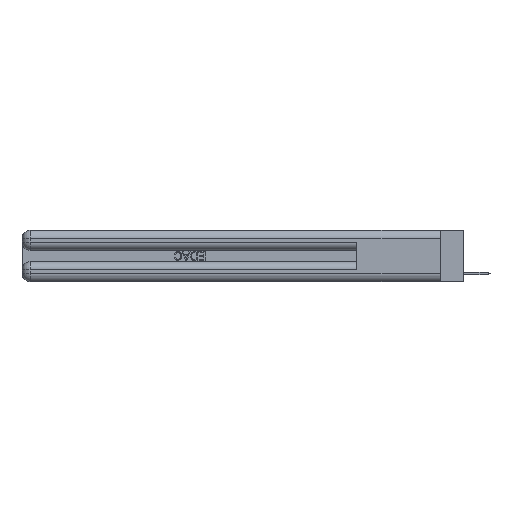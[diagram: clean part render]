
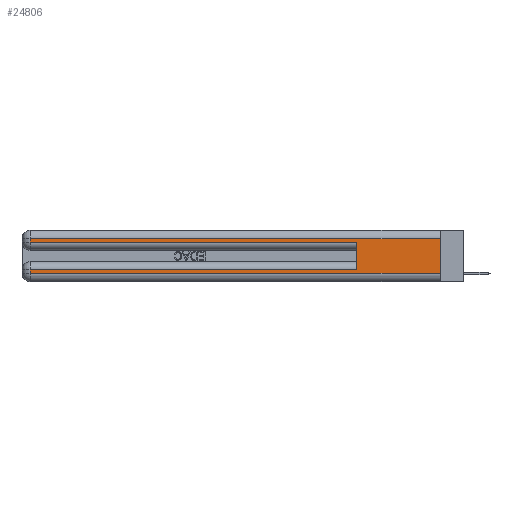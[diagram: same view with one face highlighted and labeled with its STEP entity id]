
A CAD part, left-side view. The second image highlights one B-rep face of the part: STEP entity #24806.
In plain terms, the highlighted planar face has unit normal (-1, 0, 0).
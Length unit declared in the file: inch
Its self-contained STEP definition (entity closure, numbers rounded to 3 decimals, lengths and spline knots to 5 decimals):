
#79 = VECTOR ( 'NONE', #12327, 39.37008 ) ;
#228 = DIRECTION ( 'NONE',  ( 0., 0., -1. ) ) ;
#763 = LINE ( 'NONE', #18012, #22861 ) ;
#814 = CARTESIAN_POINT ( 'NONE',  ( 0., 0.6, 0.285 ) ) ;
#931 = CARTESIAN_POINT ( 'NONE',  ( 0., 2.94, 0.31 ) ) ;
#2115 = ORIENTED_EDGE ( 'NONE', *, *, #25641, .T. ) ;
#2352 = LINE ( 'NONE', #28300, #20091 ) ;
#2500 = CARTESIAN_POINT ( 'NONE',  ( 0., 0., 0.085 ) ) ;
#2709 = ORIENTED_EDGE ( 'NONE', *, *, #18675, .T. ) ;
#3189 = DIRECTION ( 'NONE',  ( 0., 0., -1. ) ) ;
#3771 = DIRECTION ( 'NONE',  ( 0., -1., 0. ) ) ;
#4194 = LINE ( 'NONE', #7821, #12872 ) ;
#5015 = DIRECTION ( 'NONE',  ( 0., 0., -1. ) ) ;
#5407 = PLANE ( 'NONE',  #27420 ) ;
#5705 = CARTESIAN_POINT ( 'NONE',  ( 0., 0., 0.37 ) ) ;
#5815 = VERTEX_POINT ( 'NONE', #12371 ) ;
#6449 = VERTEX_POINT ( 'NONE', #814 ) ;
#6516 = EDGE_CURVE ( 'NONE', #10701, #6449, #26906, .T. ) ;
#7080 = VECTOR ( 'NONE', #3771, 39.37008 ) ;
#7821 = CARTESIAN_POINT ( 'NONE',  ( 0., 0., 0.31 ) ) ;
#8085 = EDGE_CURVE ( 'NONE', #5815, #6449, #763, .T. ) ;
#8103 = VERTEX_POINT ( 'NONE', #27344 ) ;
#8982 = CARTESIAN_POINT ( 'NONE',  ( 0., 2.94, 0.06 ) ) ;
#9684 = ORIENTED_EDGE ( 'NONE', *, *, #15189, .F. ) ;
#10701 = VERTEX_POINT ( 'NONE', #14989 ) ;
#12074 = CARTESIAN_POINT ( 'NONE',  ( 0., 0., 0.31 ) ) ;
#12327 = DIRECTION ( 'NONE',  ( 0., 0., 1. ) ) ;
#12371 = CARTESIAN_POINT ( 'NONE',  ( 0., 2.94, 0.285 ) ) ;
#12578 = DIRECTION ( 'NONE',  ( 1., 0., 0. ) ) ;
#12631 = CARTESIAN_POINT ( 'NONE',  ( 0., 0.6, 0.145 ) ) ;
#12872 = VECTOR ( 'NONE', #23879, 39.37008 ) ;
#13074 = CARTESIAN_POINT ( 'NONE',  ( 0., 0., 0.37 ) ) ;
#13651 = EDGE_CURVE ( 'NONE', #27425, #5815, #22936, .T. ) ;
#14601 = VECTOR ( 'NONE', #228, 39.37008 ) ;
#14660 = ORIENTED_EDGE ( 'NONE', *, *, #19302, .T. ) ;
#14989 = CARTESIAN_POINT ( 'NONE',  ( 0., 0.6, 0.085 ) ) ;
#15189 = EDGE_CURVE ( 'NONE', #16778, #8103, #27572, .T. ) ;
#15810 = FACE_OUTER_BOUND ( 'NONE', #24978, .T. ) ;
#16471 = LINE ( 'NONE', #17611, #7080 ) ;
#16706 = VECTOR ( 'NONE', #29312, 39.37008 ) ;
#16778 = VERTEX_POINT ( 'NONE', #12074 ) ;
#17611 = CARTESIAN_POINT ( 'NONE',  ( 0., 0., 0.06 ) ) ;
#17873 = VERTEX_POINT ( 'NONE', #18712 ) ;
#18012 = CARTESIAN_POINT ( 'NONE',  ( 0., 0., 0.285 ) ) ;
#18585 = VECTOR ( 'NONE', #25759, 39.37008 ) ;
#18675 = EDGE_CURVE ( 'NONE', #16778, #27425, #4194, .T. ) ;
#18712 = CARTESIAN_POINT ( 'NONE',  ( 0., 2.94, 0.085 ) ) ;
#19184 = ORIENTED_EDGE ( 'NONE', *, *, #8085, .T. ) ;
#19302 = EDGE_CURVE ( 'NONE', #17873, #21687, #2352, .T. ) ;
#20091 = VECTOR ( 'NONE', #5015, 39.37008 ) ;
#20131 = EDGE_CURVE ( 'NONE', #10701, #17873, #25840, .T. ) ;
#20543 = DIRECTION ( 'NONE',  ( 0., -1., 0. ) ) ;
#21687 = VERTEX_POINT ( 'NONE', #8982 ) ;
#22861 = VECTOR ( 'NONE', #20543, 39.37008 ) ;
#22936 = LINE ( 'NONE', #27991, #14601 ) ;
#23879 = DIRECTION ( 'NONE',  ( 0., 1., 0. ) ) ;
#24100 = ORIENTED_EDGE ( 'NONE', *, *, #20131, .T. ) ;
#24806 = ADVANCED_FACE ( 'NONE', ( #15810 ), #5407, .F. ) ;
#24978 = EDGE_LOOP ( 'NONE', ( #9684, #2709, #25334, #19184, #26579, #24100, #14660, #2115 ) ) ;
#25334 = ORIENTED_EDGE ( 'NONE', *, *, #13651, .T. ) ;
#25641 = EDGE_CURVE ( 'NONE', #21687, #8103, #16471, .T. ) ;
#25759 = DIRECTION ( 'NONE',  ( 0., 1., 0. ) ) ;
#25840 = LINE ( 'NONE', #2500, #18585 ) ;
#26579 = ORIENTED_EDGE ( 'NONE', *, *, #6516, .F. ) ;
#26906 = LINE ( 'NONE', #12631, #79 ) ;
#27344 = CARTESIAN_POINT ( 'NONE',  ( 0., 0., 0.06 ) ) ;
#27420 = AXIS2_PLACEMENT_3D ( 'NONE', #5705, #12578, #3189 ) ;
#27425 = VERTEX_POINT ( 'NONE', #931 ) ;
#27572 = LINE ( 'NONE', #13074, #16706 ) ;
#27991 = CARTESIAN_POINT ( 'NONE',  ( 0., 2.94, 0.37 ) ) ;
#28300 = CARTESIAN_POINT ( 'NONE',  ( 0., 2.94, 0.37 ) ) ;
#29312 = DIRECTION ( 'NONE',  ( 0., 0., -1. ) ) ;
